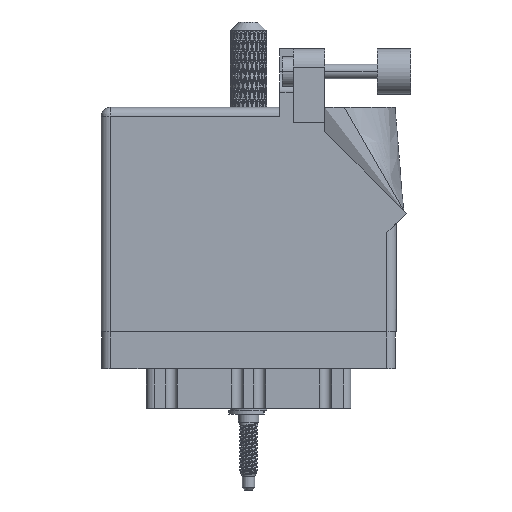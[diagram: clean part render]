
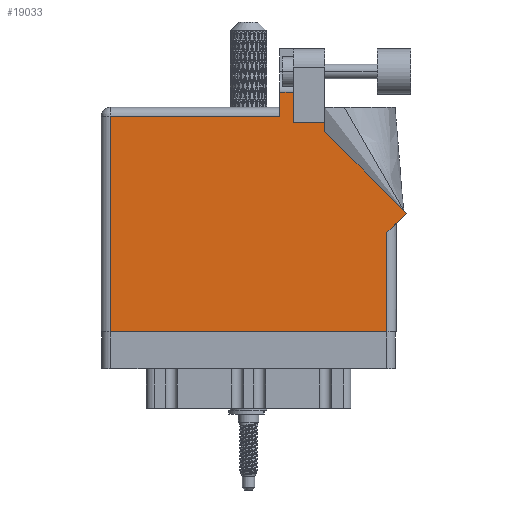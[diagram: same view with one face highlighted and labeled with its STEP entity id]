
A CAD part, front view. The second image highlights one B-rep face of the part: STEP entity #19033.
In plain terms, the highlighted face is planar.
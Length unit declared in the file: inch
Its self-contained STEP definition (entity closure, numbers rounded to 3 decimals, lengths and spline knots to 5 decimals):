
#341 = EDGE_CURVE ( 'NONE', #20807, #35189, #104618, .T. ) ;
#518 = EDGE_CURVE ( 'NONE', #86842, #8344, #934, .T. ) ;
#639 = CARTESIAN_POINT ( 'NONE',  ( 1.311, 1.6315, 0. ) ) ;
#934 = LINE ( 'NONE', #57684, #2457 ) ;
#1288 = VECTOR ( 'NONE', #43369, 39.37008 ) ;
#2457 = VECTOR ( 'NONE', #97978, 39.37008 ) ;
#2928 = VECTOR ( 'NONE', #29883, 39.37008 ) ;
#4137 = VECTOR ( 'NONE', #16058, 39.37008 ) ;
#4916 = CARTESIAN_POINT ( 'NONE',  ( 1.311, 1.43, 0. ) ) ;
#8344 = VERTEX_POINT ( 'NONE', #44549 ) ;
#10185 = VERTEX_POINT ( 'NONE', #93440 ) ;
#10438 = DIRECTION ( 'NONE',  ( 0., 0., -1. ) ) ;
#12389 = LINE ( 'NONE', #61735, #2928 ) ;
#12815 = CARTESIAN_POINT ( 'NONE',  ( 1.948, 0., 0. ) ) ;
#14765 = VECTOR ( 'NONE', #65584, 39.37008 ) ;
#15123 = LINE ( 'NONE', #54903, #68559 ) ;
#16058 = DIRECTION ( 'NONE',  ( 0., 1., 0. ) ) ;
#16778 = ORIENTED_EDGE ( 'NONE', *, *, #82626, .T. ) ;
#17556 = CARTESIAN_POINT ( 'NONE',  ( 1.217, 1.468, 0. ) ) ;
#17562 = DIRECTION ( 'NONE',  ( 0., -1., 0. ) ) ;
#19033 = ADVANCED_FACE ( 'NONE', ( #35389 ), #67752, .F. ) ;
#20807 = VERTEX_POINT ( 'NONE', #12815 ) ;
#23538 = CARTESIAN_POINT ( 'NONE',  ( 0., 1.468, 0. ) ) ;
#25026 = VECTOR ( 'NONE', #56222, 39.37008 ) ;
#25730 = ORIENTED_EDGE ( 'NONE', *, *, #50464, .T. ) ;
#27475 = CARTESIAN_POINT ( 'NONE',  ( 2.01, 0.737, 0. ) ) ;
#27507 = VERTEX_POINT ( 'NONE', #70171 ) ;
#28187 = VECTOR ( 'NONE', #37259, 39.37008 ) ;
#29883 = DIRECTION ( 'NONE',  ( 0., -1., 0. ) ) ;
#31487 = LINE ( 'NONE', #23538, #104123 ) ;
#32175 = VERTEX_POINT ( 'NONE', #37787 ) ;
#33253 = ORIENTED_EDGE ( 'NONE', *, *, #40242, .T. ) ;
#35189 = VERTEX_POINT ( 'NONE', #72150 ) ;
#35389 = FACE_OUTER_BOUND ( 'NONE', #66638, .T. ) ;
#35878 = VECTOR ( 'NONE', #17562, 39.37008 ) ;
#37259 = DIRECTION ( 'NONE',  ( 0., 1., 0. ) ) ;
#37787 = CARTESIAN_POINT ( 'NONE',  ( 1.311, 1.43, 0. ) ) ;
#39076 = CARTESIAN_POINT ( 'NONE',  ( 0.062, 0., 0. ) ) ;
#39229 = CARTESIAN_POINT ( 'NONE',  ( 2.08071, 0.80771, 0. ) ) ;
#40242 = EDGE_CURVE ( 'NONE', #52486, #10185, #31487, .T. ) ;
#41118 = CARTESIAN_POINT ( 'NONE',  ( 1.64177, 1.6315, 0. ) ) ;
#42769 = CARTESIAN_POINT ( 'NONE',  ( 0., 1.53, 0. ) ) ;
#43369 = DIRECTION ( 'NONE',  ( 0.707, 0.707, 0. ) ) ;
#44525 = EDGE_CURVE ( 'NONE', #32175, #50789, #77605, .T. ) ;
#44549 = CARTESIAN_POINT ( 'NONE',  ( 1.524, 1.43, 0. ) ) ;
#48517 = ORIENTED_EDGE ( 'NONE', *, *, #74389, .T. ) ;
#49278 = LINE ( 'NONE', #39229, #25026 ) ;
#50009 = ORIENTED_EDGE ( 'NONE', *, *, #80849, .T. ) ;
#50464 = EDGE_CURVE ( 'NONE', #64605, #20807, #15123, .T. ) ;
#50789 = VERTEX_POINT ( 'NONE', #639 ) ;
#52486 = VERTEX_POINT ( 'NONE', #17556 ) ;
#54903 = CARTESIAN_POINT ( 'NONE',  ( 0., 0., 0. ) ) ;
#56222 = DIRECTION ( 'NONE',  ( -0.707, 0.707, 0. ) ) ;
#56429 = EDGE_CURVE ( 'NONE', #68715, #86842, #49278, .T. ) ;
#57684 = CARTESIAN_POINT ( 'NONE',  ( 1.524, 1.36442, 0. ) ) ;
#59509 = VECTOR ( 'NONE', #104635, 39.37008 ) ;
#61735 = CARTESIAN_POINT ( 'NONE',  ( 0.062, 0., 0. ) ) ;
#64376 = CARTESIAN_POINT ( 'NONE',  ( 1.524, 1.43, 0. ) ) ;
#64605 = VERTEX_POINT ( 'NONE', #39076 ) ;
#65584 = DIRECTION ( 'NONE',  ( -1., 0., 0. ) ) ;
#66638 = EDGE_LOOP ( 'NONE', ( #86960, #93116, #91876, #33253, #16778, #25730, #78889, #50009, #101371, #96615, #48517 ) ) ;
#67147 = LINE ( 'NONE', #41118, #14765 ) ;
#67211 = DIRECTION ( 'NONE',  ( -1., 0., 0. ) ) ;
#67290 = LINE ( 'NONE', #27475, #1288 ) ;
#67752 = PLANE ( 'NONE',  #76565 ) ;
#68559 = VECTOR ( 'NONE', #87814, 39.37008 ) ;
#68715 = VERTEX_POINT ( 'NONE', #73600 ) ;
#70171 = CARTESIAN_POINT ( 'NONE',  ( 1.217, 1.6315, 0. ) ) ;
#72150 = CARTESIAN_POINT ( 'NONE',  ( 1.948, 0.675, 0. ) ) ;
#73600 = CARTESIAN_POINT ( 'NONE',  ( 2.08071, 0.80771, 0. ) ) ;
#74389 = EDGE_CURVE ( 'NONE', #8344, #32175, #89819, .T. ) ;
#76565 = AXIS2_PLACEMENT_3D ( 'NONE', #42769, #10438, #67211 ) ;
#77605 = LINE ( 'NONE', #4916, #28187 ) ;
#78889 = ORIENTED_EDGE ( 'NONE', *, *, #341, .T. ) ;
#79785 = DIRECTION ( 'NONE',  ( -1., 0., 0. ) ) ;
#79904 = EDGE_CURVE ( 'NONE', #50789, #27507, #67147, .T. ) ;
#80849 = EDGE_CURVE ( 'NONE', #35189, #68715, #67290, .T. ) ;
#82626 = EDGE_CURVE ( 'NONE', #10185, #64605, #12389, .T. ) ;
#86842 = VERTEX_POINT ( 'NONE', #87577 ) ;
#86960 = ORIENTED_EDGE ( 'NONE', *, *, #44525, .T. ) ;
#87577 = CARTESIAN_POINT ( 'NONE',  ( 1.524, 1.36442, 0. ) ) ;
#87814 = DIRECTION ( 'NONE',  ( 1., 0., 0. ) ) ;
#89819 = LINE ( 'NONE', #64376, #59509 ) ;
#90777 = CARTESIAN_POINT ( 'NONE',  ( 1.217, 1.53, 0. ) ) ;
#91876 = ORIENTED_EDGE ( 'NONE', *, *, #92844, .T. ) ;
#92844 = EDGE_CURVE ( 'NONE', #27507, #52486, #96620, .T. ) ;
#93116 = ORIENTED_EDGE ( 'NONE', *, *, #79904, .T. ) ;
#93440 = CARTESIAN_POINT ( 'NONE',  ( 0.062, 1.468, 0. ) ) ;
#96615 = ORIENTED_EDGE ( 'NONE', *, *, #518, .T. ) ;
#96620 = LINE ( 'NONE', #90777, #35878 ) ;
#97978 = DIRECTION ( 'NONE',  ( 0., 1., 0. ) ) ;
#98737 = CARTESIAN_POINT ( 'NONE',  ( 1.948, 0.737, 0. ) ) ;
#101371 = ORIENTED_EDGE ( 'NONE', *, *, #56429, .T. ) ;
#104123 = VECTOR ( 'NONE', #79785, 39.37008 ) ;
#104618 = LINE ( 'NONE', #98737, #4137 ) ;
#104635 = DIRECTION ( 'NONE',  ( -1., 0., 0. ) ) ;
